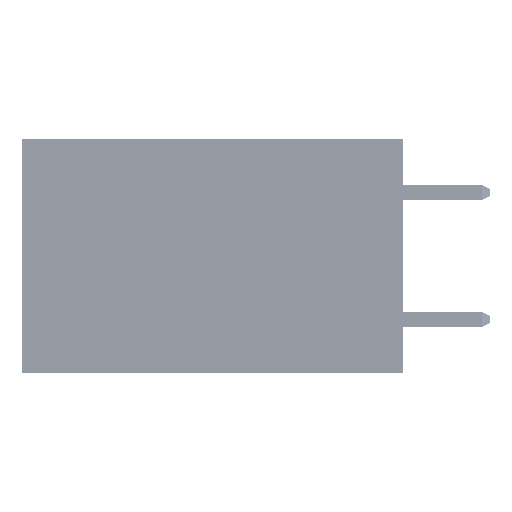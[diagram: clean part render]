
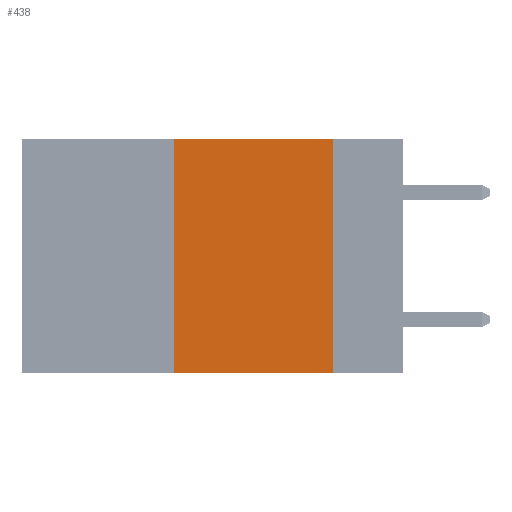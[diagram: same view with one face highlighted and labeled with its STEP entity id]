
A CAD part, left-side view. The second image highlights one B-rep face of the part: STEP entity #438.
In plain terms, the highlighted planar face has unit normal (-1, 0, 0).
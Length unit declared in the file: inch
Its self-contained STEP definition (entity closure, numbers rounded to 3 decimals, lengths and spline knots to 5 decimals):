
#438 = ADVANCED_FACE ( 'NONE', ( #26748 ), #28033, .F. ) ;
#816 = CARTESIAN_POINT ( 'NONE',  ( 0., 0.36, 0. ) ) ;
#2871 = ORIENTED_EDGE ( 'NONE', *, *, #23447, .T. ) ;
#2895 = EDGE_CURVE ( 'NONE', #8792, #9024, #10307, .T. ) ;
#5436 = CARTESIAN_POINT ( 'NONE',  ( 0., 0.36, -0.37 ) ) ;
#6013 = VECTOR ( 'NONE', #25501, 39.37008 ) ;
#6221 = DIRECTION ( 'NONE',  ( 0., 0., -1. ) ) ;
#6696 = DIRECTION ( 'NONE',  ( 1., 0., 0. ) ) ;
#7310 = LINE ( 'NONE', #49484, #6013 ) ;
#8479 = ORIENTED_EDGE ( 'NONE', *, *, #2895, .F. ) ;
#8792 = VERTEX_POINT ( 'NONE', #816 ) ;
#9024 = VERTEX_POINT ( 'NONE', #38445 ) ;
#9574 = CARTESIAN_POINT ( 'NONE',  ( 0., 0.6, -0.37 ) ) ;
#10307 = LINE ( 'NONE', #10953, #19700 ) ;
#10953 = CARTESIAN_POINT ( 'NONE',  ( 0., 0.6, 0. ) ) ;
#12035 = VECTOR ( 'NONE', #47186, 39.37008 ) ;
#12749 = VERTEX_POINT ( 'NONE', #47421 ) ;
#13568 = DIRECTION ( 'NONE',  ( 0., -1., 0. ) ) ;
#15110 = CARTESIAN_POINT ( 'NONE',  ( 0., 0.11, 0. ) ) ;
#15869 = CARTESIAN_POINT ( 'NONE',  ( 0., 0.6, 0. ) ) ;
#18554 = LINE ( 'NONE', #9574, #38655 ) ;
#19700 = VECTOR ( 'NONE', #51037, 39.37008 ) ;
#23447 = EDGE_CURVE ( 'NONE', #29735, #12749, #18554, .T. ) ;
#25501 = DIRECTION ( 'NONE',  ( 0., 0., 1. ) ) ;
#25832 = EDGE_CURVE ( 'NONE', #9024, #12749, #34590, .T. ) ;
#26748 = FACE_OUTER_BOUND ( 'NONE', #51045, .T. ) ;
#28033 = PLANE ( 'NONE',  #38947 ) ;
#29735 = VERTEX_POINT ( 'NONE', #5436 ) ;
#34590 = LINE ( 'NONE', #15110, #12035 ) ;
#38445 = CARTESIAN_POINT ( 'NONE',  ( 0., 0.11, 0. ) ) ;
#38655 = VECTOR ( 'NONE', #13568, 39.37008 ) ;
#38947 = AXIS2_PLACEMENT_3D ( 'NONE', #15869, #6696, #6221 ) ;
#43381 = ORIENTED_EDGE ( 'NONE', *, *, #49543, .F. ) ;
#47186 = DIRECTION ( 'NONE',  ( 0., 0., -1. ) ) ;
#47421 = CARTESIAN_POINT ( 'NONE',  ( 0., 0.11, -0.37 ) ) ;
#48898 = ORIENTED_EDGE ( 'NONE', *, *, #25832, .F. ) ;
#49484 = CARTESIAN_POINT ( 'NONE',  ( 0., 0.36, 0. ) ) ;
#49543 = EDGE_CURVE ( 'NONE', #29735, #8792, #7310, .T. ) ;
#51037 = DIRECTION ( 'NONE',  ( 0., -1., 0. ) ) ;
#51045 = EDGE_LOOP ( 'NONE', ( #48898, #8479, #43381, #2871 ) ) ;
